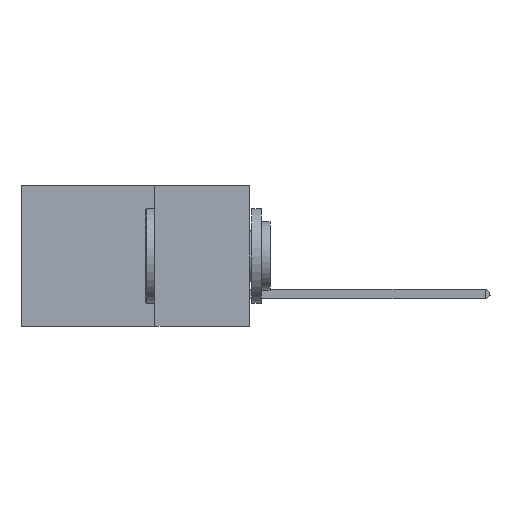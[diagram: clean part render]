
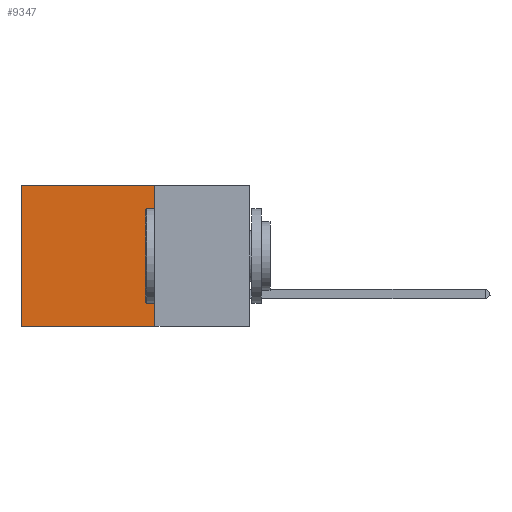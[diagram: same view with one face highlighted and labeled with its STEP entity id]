
A CAD part, left-side view. The second image highlights one B-rep face of the part: STEP entity #9347.
In plain terms, the highlighted planar face has unit normal (-1, 0, 0).
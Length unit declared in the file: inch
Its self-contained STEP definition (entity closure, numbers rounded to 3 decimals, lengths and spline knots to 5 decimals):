
#1525 = LINE ( 'NONE', #30690, #13613 ) ;
#1819 = ORIENTED_EDGE ( 'NONE', *, *, #28256, .F. ) ;
#1925 = DIRECTION ( 'NONE',  ( 0., 0., -1. ) ) ;
#2427 = AXIS2_PLACEMENT_3D ( 'NONE', #16967, #45923, #1925 ) ;
#2948 = VERTEX_POINT ( 'NONE', #22649 ) ;
#3555 = LINE ( 'NONE', #4041, #13368 ) ;
#3869 = VERTEX_POINT ( 'NONE', #5184 ) ;
#4041 = CARTESIAN_POINT ( 'NONE',  ( 0.2875, 0.25, 0. ) ) ;
#4704 = VERTEX_POINT ( 'NONE', #22162 ) ;
#5184 = CARTESIAN_POINT ( 'NONE',  ( 0.2875, 0.25, -0.37 ) ) ;
#9347 = ADVANCED_FACE ( 'NONE', ( #28588 ), #27454, .F. ) ;
#13368 = VECTOR ( 'NONE', #29838, 39.37008 ) ;
#13613 = VECTOR ( 'NONE', #45926, 39.37008 ) ;
#15181 = EDGE_LOOP ( 'NONE', ( #45975, #1819, #21372, #39516 ) ) ;
#16967 = CARTESIAN_POINT ( 'NONE',  ( 0.2875, 0.25, 0. ) ) ;
#17651 = VECTOR ( 'NONE', #19418, 39.37008 ) ;
#19418 = DIRECTION ( 'NONE',  ( 0., 1., 0. ) ) ;
#21372 = ORIENTED_EDGE ( 'NONE', *, *, #39204, .F. ) ;
#22162 = CARTESIAN_POINT ( 'NONE',  ( 0.2875, 0.25, 0. ) ) ;
#22649 = CARTESIAN_POINT ( 'NONE',  ( 0.2875, 0.6, -0.37 ) ) ;
#23659 = CARTESIAN_POINT ( 'NONE',  ( 0.2875, 0.6, 0. ) ) ;
#27454 = PLANE ( 'NONE',  #2427 ) ;
#27471 = LINE ( 'NONE', #45758, #17651 ) ;
#28256 = EDGE_CURVE ( 'NONE', #3869, #2948, #27471, .T. ) ;
#28588 = FACE_OUTER_BOUND ( 'NONE', #15181, .T. ) ;
#29838 = DIRECTION ( 'NONE',  ( 0., 0., -1. ) ) ;
#30690 = CARTESIAN_POINT ( 'NONE',  ( 0.2875, 0.6, 0. ) ) ;
#34092 = VERTEX_POINT ( 'NONE', #23659 ) ;
#34140 = CARTESIAN_POINT ( 'NONE',  ( 0.2875, 0.25, 0. ) ) ;
#37000 = EDGE_CURVE ( 'NONE', #34092, #2948, #1525, .T. ) ;
#37436 = VECTOR ( 'NONE', #38737, 39.37008 ) ;
#38737 = DIRECTION ( 'NONE',  ( 0., 1., 0. ) ) ;
#39204 = EDGE_CURVE ( 'NONE', #4704, #3869, #3555, .T. ) ;
#39516 = ORIENTED_EDGE ( 'NONE', *, *, #46983, .T. ) ;
#43740 = LINE ( 'NONE', #34140, #37436 ) ;
#45758 = CARTESIAN_POINT ( 'NONE',  ( 0.2875, 0.25, -0.37 ) ) ;
#45923 = DIRECTION ( 'NONE',  ( 1., 0., 0. ) ) ;
#45926 = DIRECTION ( 'NONE',  ( 0., 0., -1. ) ) ;
#45975 = ORIENTED_EDGE ( 'NONE', *, *, #37000, .T. ) ;
#46983 = EDGE_CURVE ( 'NONE', #4704, #34092, #43740, .T. ) ;
